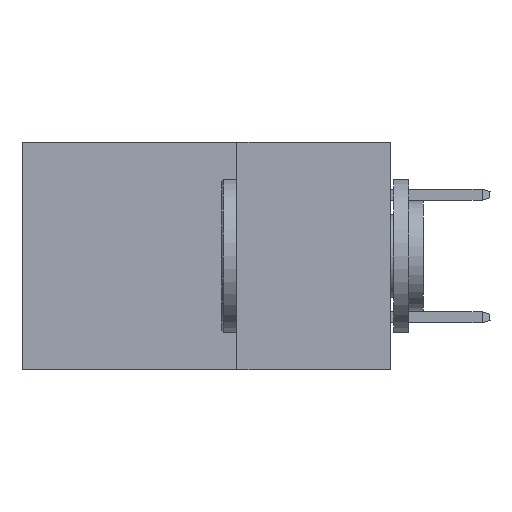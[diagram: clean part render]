
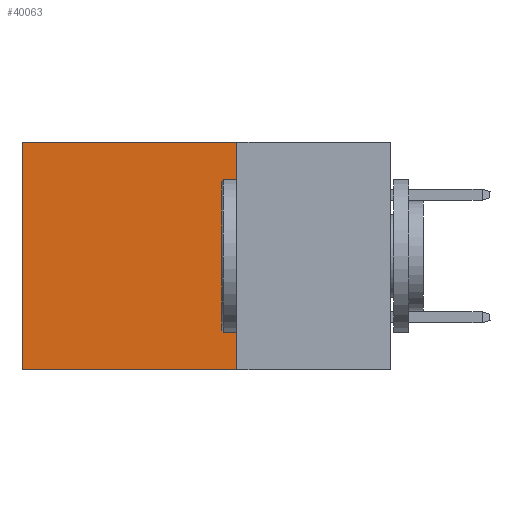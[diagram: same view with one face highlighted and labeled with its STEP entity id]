
A CAD part, left-side view. The second image highlights one B-rep face of the part: STEP entity #40063.
In plain terms, the highlighted planar face has unit normal (-1, 0, 0).
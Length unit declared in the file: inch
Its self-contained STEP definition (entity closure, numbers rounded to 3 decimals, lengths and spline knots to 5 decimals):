
#140 = DIRECTION ( 'NONE',  ( 0., 0., -1. ) ) ;
#1122 = LINE ( 'NONE', #14100, #2256 ) ;
#2224 = PLANE ( 'NONE',  #19210 ) ;
#2256 = VECTOR ( 'NONE', #17628, 39.37008 ) ;
#2469 = CARTESIAN_POINT ( 'NONE',  ( 0.2875, 0.6, -0.37 ) ) ;
#3606 = VECTOR ( 'NONE', #140, 39.37008 ) ;
#5820 = VERTEX_POINT ( 'NONE', #33204 ) ;
#8997 = EDGE_CURVE ( 'NONE', #5820, #43613, #40316, .T. ) ;
#9164 = DIRECTION ( 'NONE',  ( 0., 1., 0. ) ) ;
#12838 = DIRECTION ( 'NONE',  ( 1., 0., 0. ) ) ;
#14100 = CARTESIAN_POINT ( 'NONE',  ( 0.2875, 0.25, 0. ) ) ;
#15542 = ORIENTED_EDGE ( 'NONE', *, *, #22632, .T. ) ;
#16396 = CARTESIAN_POINT ( 'NONE',  ( 0.2875, 0.25, 0. ) ) ;
#17628 = DIRECTION ( 'NONE',  ( 0., 1., 0. ) ) ;
#19132 = ORIENTED_EDGE ( 'NONE', *, *, #8997, .F. ) ;
#19210 = AXIS2_PLACEMENT_3D ( 'NONE', #33758, #12838, #37241 ) ;
#20484 = EDGE_CURVE ( 'NONE', #31823, #27968, #1122, .T. ) ;
#21793 = VECTOR ( 'NONE', #9164, 39.37008 ) ;
#21838 = VECTOR ( 'NONE', #39799, 39.37008 ) ;
#22632 = EDGE_CURVE ( 'NONE', #27968, #43613, #32187, .T. ) ;
#24738 = CARTESIAN_POINT ( 'NONE',  ( 0.2875, 0.25, 0. ) ) ;
#27158 = ORIENTED_EDGE ( 'NONE', *, *, #29241, .F. ) ;
#27968 = VERTEX_POINT ( 'NONE', #42404 ) ;
#29241 = EDGE_CURVE ( 'NONE', #31823, #5820, #40843, .T. ) ;
#31823 = VERTEX_POINT ( 'NONE', #16396 ) ;
#32187 = LINE ( 'NONE', #32787, #21838 ) ;
#32306 = ORIENTED_EDGE ( 'NONE', *, *, #20484, .T. ) ;
#32787 = CARTESIAN_POINT ( 'NONE',  ( 0.2875, 0.6, 0. ) ) ;
#33048 = EDGE_LOOP ( 'NONE', ( #15542, #19132, #27158, #32306 ) ) ;
#33204 = CARTESIAN_POINT ( 'NONE',  ( 0.2875, 0.25, -0.37 ) ) ;
#33758 = CARTESIAN_POINT ( 'NONE',  ( 0.2875, 0.25, 0. ) ) ;
#37241 = DIRECTION ( 'NONE',  ( 0., 0., -1. ) ) ;
#39087 = FACE_OUTER_BOUND ( 'NONE', #33048, .T. ) ;
#39799 = DIRECTION ( 'NONE',  ( 0., 0., -1. ) ) ;
#40063 = ADVANCED_FACE ( 'NONE', ( #39087 ), #2224, .F. ) ;
#40316 = LINE ( 'NONE', #44002, #21793 ) ;
#40843 = LINE ( 'NONE', #24738, #3606 ) ;
#42404 = CARTESIAN_POINT ( 'NONE',  ( 0.2875, 0.6, 0. ) ) ;
#43613 = VERTEX_POINT ( 'NONE', #2469 ) ;
#44002 = CARTESIAN_POINT ( 'NONE',  ( 0.2875, 0.25, -0.37 ) ) ;
